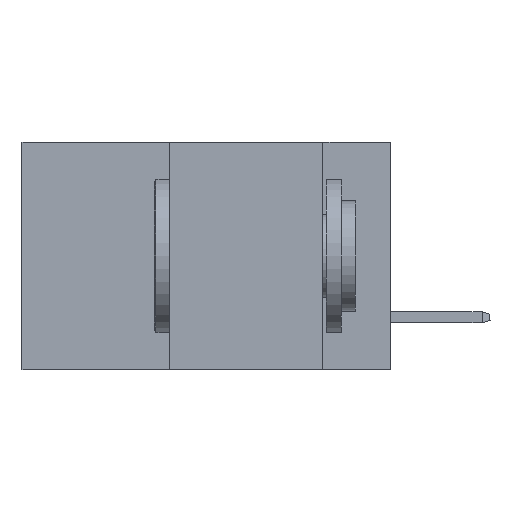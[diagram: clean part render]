
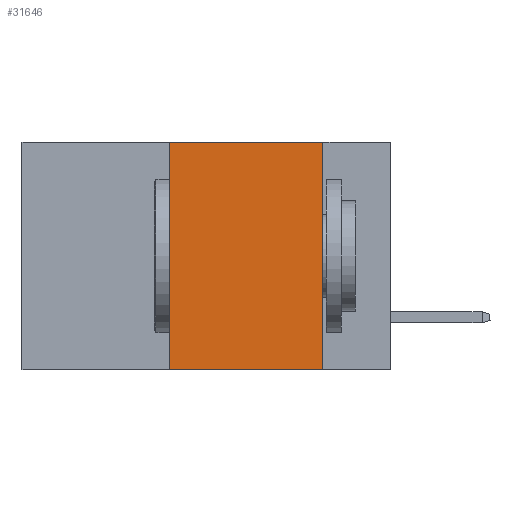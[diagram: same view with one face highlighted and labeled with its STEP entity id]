
A CAD part, left-side view. The second image highlights one B-rep face of the part: STEP entity #31646.
In plain terms, the highlighted planar face has unit normal (-1, 0, 0).
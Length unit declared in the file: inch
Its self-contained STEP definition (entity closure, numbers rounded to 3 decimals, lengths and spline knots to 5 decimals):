
#178 = CARTESIAN_POINT ( 'NONE',  ( 0., 0.36, 0. ) ) ;
#734 = DIRECTION ( 'NONE',  ( 0., 0., -1. ) ) ;
#2081 = EDGE_CURVE ( 'NONE', #11237, #35377, #8277, .T. ) ;
#4371 = ORIENTED_EDGE ( 'NONE', *, *, #15437, .T. ) ;
#5179 = VECTOR ( 'NONE', #45926, 39.37008 ) ;
#6178 = CARTESIAN_POINT ( 'NONE',  ( 0., 0.11, -0.37 ) ) ;
#6472 = LINE ( 'NONE', #26447, #5179 ) ;
#6504 = ORIENTED_EDGE ( 'NONE', *, *, #31368, .F. ) ;
#7768 = VECTOR ( 'NONE', #46080, 39.37008 ) ;
#8277 = LINE ( 'NONE', #178, #48936 ) ;
#8764 = EDGE_CURVE ( 'NONE', #35377, #26081, #6472, .T. ) ;
#9930 = CARTESIAN_POINT ( 'NONE',  ( 0., 0.11, 0. ) ) ;
#10066 = CARTESIAN_POINT ( 'NONE',  ( 0., 0.11, 0. ) ) ;
#11237 = VERTEX_POINT ( 'NONE', #16138 ) ;
#14193 = DIRECTION ( 'NONE',  ( 0., 0., -1. ) ) ;
#15334 = VERTEX_POINT ( 'NONE', #6178 ) ;
#15437 = EDGE_CURVE ( 'NONE', #11237, #15334, #34934, .T. ) ;
#15933 = PLANE ( 'NONE',  #43493 ) ;
#16138 = CARTESIAN_POINT ( 'NONE',  ( 0., 0.36, -0.37 ) ) ;
#20233 = CARTESIAN_POINT ( 'NONE',  ( 0., 0.6, 0. ) ) ;
#26081 = VERTEX_POINT ( 'NONE', #10066 ) ;
#26447 = CARTESIAN_POINT ( 'NONE',  ( 0., 0.6, 0. ) ) ;
#28355 = EDGE_LOOP ( 'NONE', ( #6504, #50858, #32474, #4371 ) ) ;
#31368 = EDGE_CURVE ( 'NONE', #26081, #15334, #44041, .T. ) ;
#31646 = ADVANCED_FACE ( 'NONE', ( #47127 ), #15933, .F. ) ;
#31716 = DIRECTION ( 'NONE',  ( 0., 0., 1. ) ) ;
#32474 = ORIENTED_EDGE ( 'NONE', *, *, #2081, .F. ) ;
#33563 = VECTOR ( 'NONE', #14193, 39.37008 ) ;
#34934 = LINE ( 'NONE', #49894, #7768 ) ;
#35377 = VERTEX_POINT ( 'NONE', #37064 ) ;
#37064 = CARTESIAN_POINT ( 'NONE',  ( 0., 0.36, 0. ) ) ;
#40096 = DIRECTION ( 'NONE',  ( 1., 0., 0. ) ) ;
#43493 = AXIS2_PLACEMENT_3D ( 'NONE', #20233, #40096, #734 ) ;
#44041 = LINE ( 'NONE', #9930, #33563 ) ;
#45926 = DIRECTION ( 'NONE',  ( 0., -1., 0. ) ) ;
#46080 = DIRECTION ( 'NONE',  ( 0., -1., 0. ) ) ;
#47127 = FACE_OUTER_BOUND ( 'NONE', #28355, .T. ) ;
#48936 = VECTOR ( 'NONE', #31716, 39.37008 ) ;
#49894 = CARTESIAN_POINT ( 'NONE',  ( 0., 0.6, -0.37 ) ) ;
#50858 = ORIENTED_EDGE ( 'NONE', *, *, #8764, .F. ) ;
